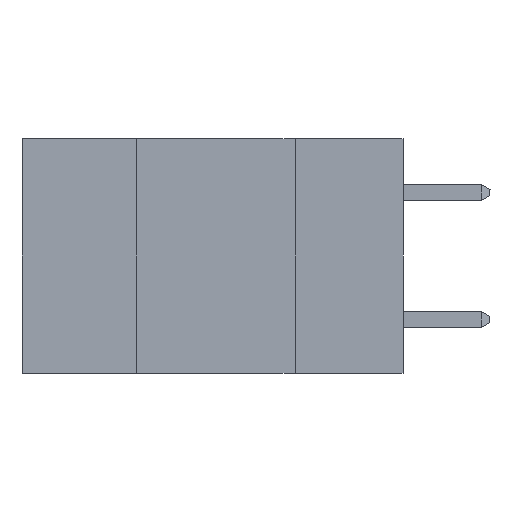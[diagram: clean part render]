
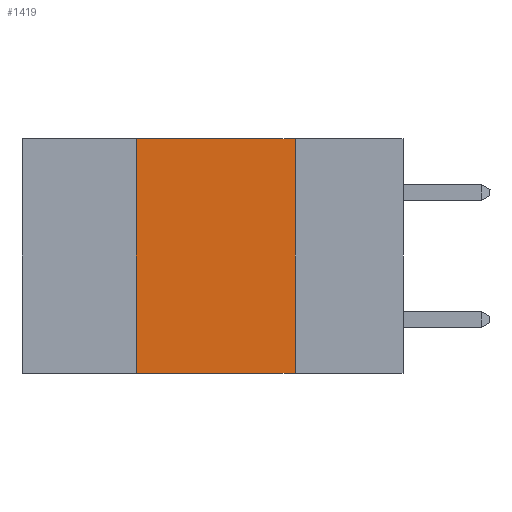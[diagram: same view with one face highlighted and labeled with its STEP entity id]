
A CAD part, left-side view. The second image highlights one B-rep face of the part: STEP entity #1419.
In plain terms, the highlighted planar face has unit normal (-1, 0, 0).
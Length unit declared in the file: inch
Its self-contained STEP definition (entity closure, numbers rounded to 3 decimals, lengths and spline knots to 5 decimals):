
#305 = VECTOR ( 'NONE', #4936, 39.37008 ) ;
#489 = ORIENTED_EDGE ( 'NONE', *, *, #6366, .F. ) ;
#1419 = ADVANCED_FACE ( 'NONE', ( #11687 ), #7217, .F. ) ;
#2302 = VERTEX_POINT ( 'NONE', #13039 ) ;
#2571 = CARTESIAN_POINT ( 'NONE',  ( 0., 0.17, -0.37 ) ) ;
#3359 = LINE ( 'NONE', #9456, #305 ) ;
#4456 = CARTESIAN_POINT ( 'NONE',  ( 0., 0.6, 0. ) ) ;
#4662 = EDGE_CURVE ( 'NONE', #2302, #5408, #9275, .T. ) ;
#4794 = CARTESIAN_POINT ( 'NONE',  ( 0., 0.17, 0. ) ) ;
#4936 = DIRECTION ( 'NONE',  ( 0., -1., 0. ) ) ;
#5408 = VERTEX_POINT ( 'NONE', #2571 ) ;
#5449 = VECTOR ( 'NONE', #8150, 39.37008 ) ;
#5539 = ORIENTED_EDGE ( 'NONE', *, *, #11859, .T. ) ;
#5818 = CARTESIAN_POINT ( 'NONE',  ( 0., 0.42, 0. ) ) ;
#5935 = AXIS2_PLACEMENT_3D ( 'NONE', #8388, #8422, #14361 ) ;
#6228 = VECTOR ( 'NONE', #12817, 39.37008 ) ;
#6366 = EDGE_CURVE ( 'NONE', #8455, #2302, #10669, .T. ) ;
#6489 = EDGE_CURVE ( 'NONE', #13768, #8455, #8528, .T. ) ;
#7217 = PLANE ( 'NONE',  #5935 ) ;
#8150 = DIRECTION ( 'NONE',  ( 0., 0., 1. ) ) ;
#8388 = CARTESIAN_POINT ( 'NONE',  ( 0., 0.6, 0. ) ) ;
#8422 = DIRECTION ( 'NONE',  ( 1., 0., 0. ) ) ;
#8455 = VERTEX_POINT ( 'NONE', #5818 ) ;
#8528 = LINE ( 'NONE', #12724, #5449 ) ;
#9275 = LINE ( 'NONE', #4794, #6228 ) ;
#9341 = ORIENTED_EDGE ( 'NONE', *, *, #4662, .F. ) ;
#9456 = CARTESIAN_POINT ( 'NONE',  ( 0., 0.6, -0.37 ) ) ;
#9741 = CARTESIAN_POINT ( 'NONE',  ( 0., 0.42, -0.37 ) ) ;
#10298 = VECTOR ( 'NONE', #12485, 39.37008 ) ;
#10669 = LINE ( 'NONE', #4456, #10298 ) ;
#11413 = ORIENTED_EDGE ( 'NONE', *, *, #6489, .F. ) ;
#11687 = FACE_OUTER_BOUND ( 'NONE', #12212, .T. ) ;
#11859 = EDGE_CURVE ( 'NONE', #13768, #5408, #3359, .T. ) ;
#12212 = EDGE_LOOP ( 'NONE', ( #9341, #489, #11413, #5539 ) ) ;
#12485 = DIRECTION ( 'NONE',  ( 0., -1., 0. ) ) ;
#12724 = CARTESIAN_POINT ( 'NONE',  ( 0., 0.42, 0. ) ) ;
#12817 = DIRECTION ( 'NONE',  ( 0., 0., -1. ) ) ;
#13039 = CARTESIAN_POINT ( 'NONE',  ( 0., 0.17, 0. ) ) ;
#13768 = VERTEX_POINT ( 'NONE', #9741 ) ;
#14361 = DIRECTION ( 'NONE',  ( 0., 0., -1. ) ) ;
